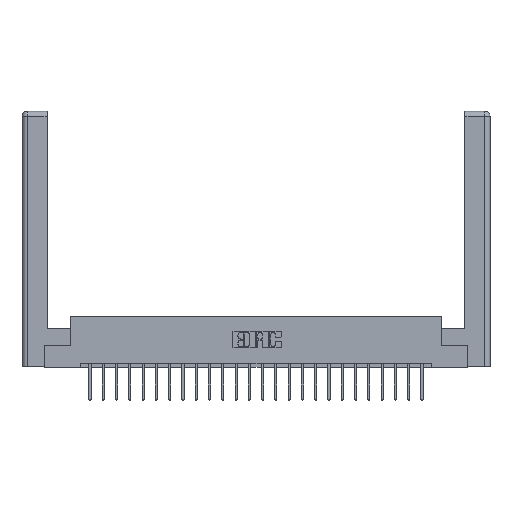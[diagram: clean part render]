
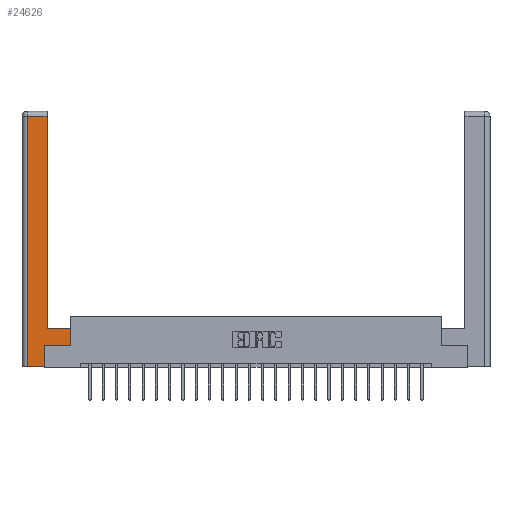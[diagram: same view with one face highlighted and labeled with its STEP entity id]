
A CAD part, top view. The second image highlights one B-rep face of the part: STEP entity #24626.
In plain terms, the highlighted planar face has unit normal (0, 0, 1).
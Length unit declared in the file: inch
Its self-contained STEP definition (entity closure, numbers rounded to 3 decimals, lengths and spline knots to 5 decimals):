
#268 = CARTESIAN_POINT ( 'NONE',  ( 0.295, 0.45, 0. ) ) ;
#543 = LINE ( 'NONE', #18212, #2664 ) ;
#1427 = ORIENTED_EDGE ( 'NONE', *, *, #2341, .T. ) ;
#1500 = EDGE_CURVE ( 'NONE', #13312, #4465, #21368, .T. ) ;
#1853 = LINE ( 'NONE', #24520, #16021 ) ;
#2341 = EDGE_CURVE ( 'NONE', #10147, #19009, #9066, .T. ) ;
#2649 = CARTESIAN_POINT ( 'NONE',  ( 0.295, 2.94, 0. ) ) ;
#2664 = VECTOR ( 'NONE', #20384, 39.37008 ) ;
#3208 = ORIENTED_EDGE ( 'NONE', *, *, #5095, .T. ) ;
#3516 = DIRECTION ( 'NONE',  ( 1., 0., 0. ) ) ;
#4285 = EDGE_CURVE ( 'NONE', #9493, #18449, #7421, .T. ) ;
#4465 = VERTEX_POINT ( 'NONE', #17192 ) ;
#4870 = ORIENTED_EDGE ( 'NONE', *, *, #4285, .T. ) ;
#4892 = DIRECTION ( 'NONE',  ( -1., 0., 0. ) ) ;
#4894 = DIRECTION ( 'NONE',  ( -1., 0., 0. ) ) ;
#5095 = EDGE_CURVE ( 'NONE', #20068, #13312, #24821, .T. ) ;
#6424 = AXIS2_PLACEMENT_3D ( 'NONE', #23985, #10631, #4894 ) ;
#7073 = CARTESIAN_POINT ( 'NONE',  ( 0.565, 0.245, 0. ) ) ;
#7300 = CARTESIAN_POINT ( 'NONE',  ( 0.265, 0., 0. ) ) ;
#7421 = LINE ( 'NONE', #7073, #17074 ) ;
#7599 = CARTESIAN_POINT ( 'NONE',  ( 0.295, 0.45, 0. ) ) ;
#8208 = LINE ( 'NONE', #7300, #14216 ) ;
#8214 = DIRECTION ( 'NONE',  ( -1., 0., 0. ) ) ;
#8233 = VECTOR ( 'NONE', #8878, 39.37008 ) ;
#8856 = EDGE_LOOP ( 'NONE', ( #17844, #3208, #24768, #20650, #20700, #4870, #14501, #1427 ) ) ;
#8878 = DIRECTION ( 'NONE',  ( 0., 1., 0. ) ) ;
#9010 = DIRECTION ( 'NONE',  ( 0., 1., 0. ) ) ;
#9052 = VECTOR ( 'NONE', #13400, 39.37008 ) ;
#9066 = LINE ( 'NONE', #268, #9962 ) ;
#9493 = VERTEX_POINT ( 'NONE', #20026 ) ;
#9962 = VECTOR ( 'NONE', #8214, 39.37008 ) ;
#10147 = VERTEX_POINT ( 'NONE', #22323 ) ;
#10541 = PLANE ( 'NONE',  #6424 ) ;
#10627 = CARTESIAN_POINT ( 'NONE',  ( 0.0615, 2.94, 0. ) ) ;
#10631 = DIRECTION ( 'NONE',  ( 0., 0., -1. ) ) ;
#11459 = EDGE_CURVE ( 'NONE', #12954, #9493, #543, .T. ) ;
#12954 = VERTEX_POINT ( 'NONE', #16340 ) ;
#13312 = VERTEX_POINT ( 'NONE', #21653 ) ;
#13400 = DIRECTION ( 'NONE',  ( 0., -1., 0. ) ) ;
#13611 = CARTESIAN_POINT ( 'NONE',  ( 0.565, 0.245, 0. ) ) ;
#14216 = VECTOR ( 'NONE', #3516, 39.37008 ) ;
#14501 = ORIENTED_EDGE ( 'NONE', *, *, #15326, .T. ) ;
#14605 = CARTESIAN_POINT ( 'NONE',  ( 0.565, 0.45, 0. ) ) ;
#15326 = EDGE_CURVE ( 'NONE', #18449, #10147, #24140, .T. ) ;
#15836 = EDGE_CURVE ( 'NONE', #19009, #20068, #1853, .T. ) ;
#15842 = EDGE_CURVE ( 'NONE', #4465, #12954, #8208, .T. ) ;
#16021 = VECTOR ( 'NONE', #9010, 39.37008 ) ;
#16340 = CARTESIAN_POINT ( 'NONE',  ( 0.265, 0., 0. ) ) ;
#17074 = VECTOR ( 'NONE', #20864, 39.37008 ) ;
#17192 = CARTESIAN_POINT ( 'NONE',  ( 0.0615, 0., 0. ) ) ;
#17844 = ORIENTED_EDGE ( 'NONE', *, *, #15836, .T. ) ;
#18212 = CARTESIAN_POINT ( 'NONE',  ( 0.265, 0.245, 0. ) ) ;
#18449 = VERTEX_POINT ( 'NONE', #13611 ) ;
#19009 = VERTEX_POINT ( 'NONE', #7599 ) ;
#19016 = CARTESIAN_POINT ( 'NONE',  ( 0.0615, 0., 0. ) ) ;
#19136 = VECTOR ( 'NONE', #4892, 39.37008 ) ;
#20026 = CARTESIAN_POINT ( 'NONE',  ( 0.265, 0.245, 0. ) ) ;
#20068 = VERTEX_POINT ( 'NONE', #2649 ) ;
#20384 = DIRECTION ( 'NONE',  ( 0., 1., 0. ) ) ;
#20650 = ORIENTED_EDGE ( 'NONE', *, *, #15842, .T. ) ;
#20700 = ORIENTED_EDGE ( 'NONE', *, *, #11459, .T. ) ;
#20864 = DIRECTION ( 'NONE',  ( 1., 0., 0. ) ) ;
#21368 = LINE ( 'NONE', #19016, #9052 ) ;
#21653 = CARTESIAN_POINT ( 'NONE',  ( 0.0615, 2.94, 0. ) ) ;
#22323 = CARTESIAN_POINT ( 'NONE',  ( 0.565, 0.45, 0. ) ) ;
#23985 = CARTESIAN_POINT ( 'NONE',  ( 0., 0., 0. ) ) ;
#24140 = LINE ( 'NONE', #14605, #8233 ) ;
#24520 = CARTESIAN_POINT ( 'NONE',  ( 0.295, 3., 0. ) ) ;
#24626 = ADVANCED_FACE ( 'NONE', ( #24743 ), #10541, .F. ) ;
#24743 = FACE_OUTER_BOUND ( 'NONE', #8856, .T. ) ;
#24768 = ORIENTED_EDGE ( 'NONE', *, *, #1500, .T. ) ;
#24821 = LINE ( 'NONE', #10627, #19136 ) ;
